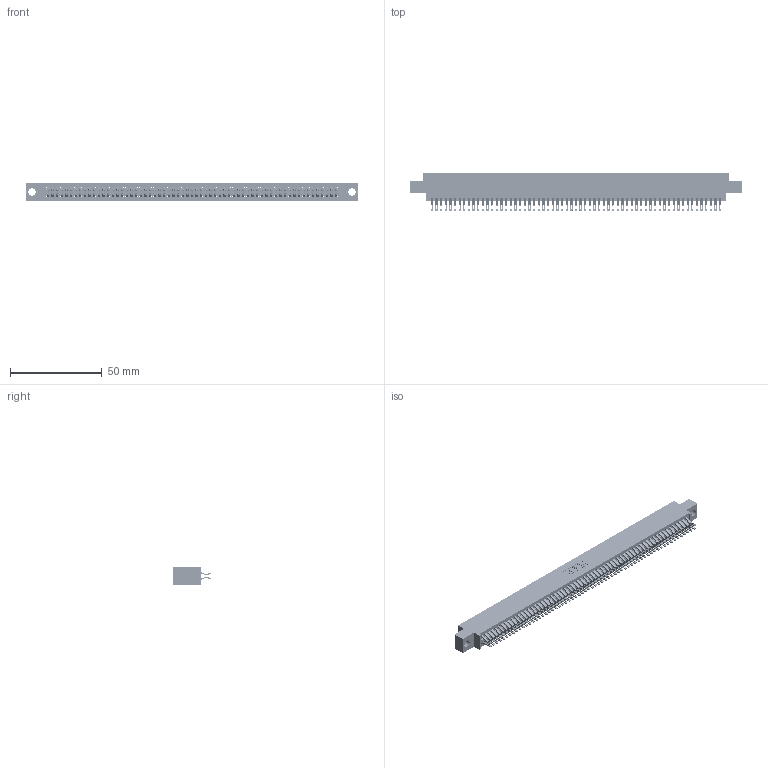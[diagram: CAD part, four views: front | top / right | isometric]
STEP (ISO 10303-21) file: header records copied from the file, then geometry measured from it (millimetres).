
FILE_DESCRIPTION (( 'STEP AP203' ), '1' );
FILE_NAME ('345-126-555-804.STEP', '2018-10-19T17:17:32', ( '' ), ( '' ), 'SwSTEP 2.0', 'SolidWorks 2016', '' );
FILE_SCHEMA (( 'CONFIG_CONTROL_DESIGN' ));
Length unit declared in the file: inch
Products named in the file (3): 345-292-001_555 Tail; 345 Part_0.170 Offset - 0.156 Dia-TH; 345-126-555-804
Assembly tree (127 placements, depth 2):
  345-126-555-804
    345 Part_0.170 Offset - 0.156 Dia-TH
    345-292-001_555 Tail  x126
Bounding box: 181.23 x 21.13 x 9.4 mm (x, y, z)
Volume: 17963.9 mm3; surface area: 28190.2 mm2
Topology: 127 solids, 127 shells, 7186 faces, 22655 edges, 15102 vertices
Faces by surface type: plane 3990, cylinder 3196
Entity records: 47065 total; most frequent: CARTESIAN_POINT 7906, ORIENTED_EDGE 7810, DIRECTION 6913, EDGE_CURVE 3905, LINE 3501, VECTOR 3501, VERTEX_POINT 2602, AXIS2_PLACEMENT_3D 1706
